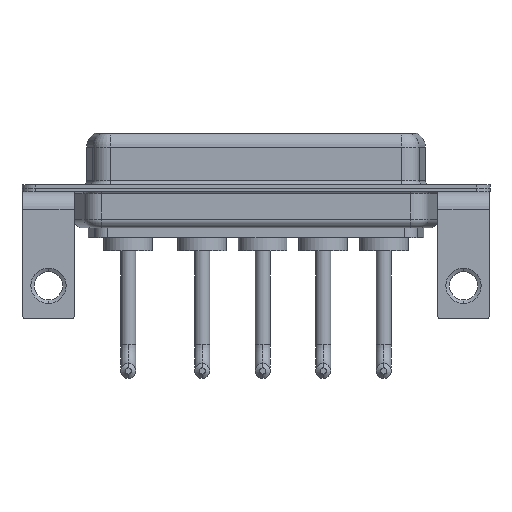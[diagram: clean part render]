
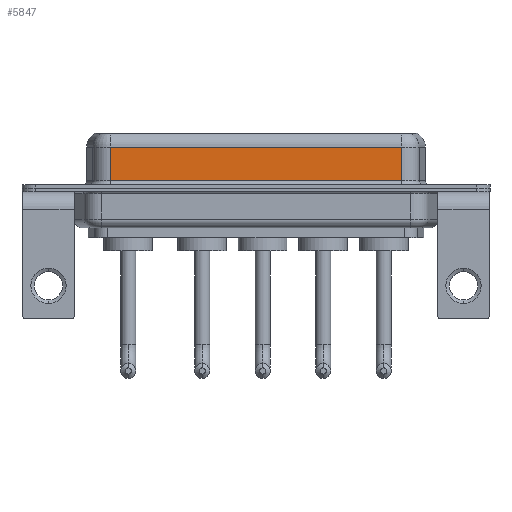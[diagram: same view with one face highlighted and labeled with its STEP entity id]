
A CAD part, front view. The second image highlights one B-rep face of the part: STEP entity #5847.
In plain terms, the highlighted planar face has unit normal (0, -1, 0).
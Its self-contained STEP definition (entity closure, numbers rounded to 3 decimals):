
#731 = CARTESIAN_POINT ( 'NONE',  ( 7.013, -3.95, 6.4 ) ) ;
#1156 = CARTESIAN_POINT ( 'NONE',  ( 40.037, -3.95, 6.4 ) ) ;
#1762 = CARTESIAN_POINT ( 'NONE',  ( 40.037, -3.95, 0.9 ) ) ;
#1887 = VECTOR ( 'NONE', #12253, 1000. ) ;
#1921 = CARTESIAN_POINT ( 'NONE',  ( 40.037, -3.95, 0.9 ) ) ;
#2321 = ORIENTED_EDGE ( 'NONE', *, *, #8391, .T. ) ;
#3272 = ORIENTED_EDGE ( 'NONE', *, *, #5163, .T. ) ;
#3285 = VERTEX_POINT ( 'NONE', #9880 ) ;
#3737 = LINE ( 'NONE', #1762, #1887 ) ;
#3812 = LINE ( 'NONE', #731, #10979 ) ;
#5163 = EDGE_CURVE ( 'NONE', #3285, #8501, #3737, .T. ) ;
#5331 = DIRECTION ( 'NONE',  ( 0., 1., 0. ) ) ;
#5847 = ADVANCED_FACE ( 'NONE', ( #6376 ), #9609, .F. ) ;
#5877 = CARTESIAN_POINT ( 'NONE',  ( 40.037, -3.95, 6.4 ) ) ;
#5925 = ORIENTED_EDGE ( 'NONE', *, *, #10108, .F. ) ;
#6376 = FACE_OUTER_BOUND ( 'NONE', #12402, .T. ) ;
#7046 = LINE ( 'NONE', #10032, #8157 ) ;
#7279 = VERTEX_POINT ( 'NONE', #11904 ) ;
#7931 = DIRECTION ( 'NONE',  ( 0., 0., -1. ) ) ;
#8157 = VECTOR ( 'NONE', #10154, 1000. ) ;
#8391 = EDGE_CURVE ( 'NONE', #7279, #12437, #7046, .T. ) ;
#8501 = VERTEX_POINT ( 'NONE', #1921 ) ;
#8765 = EDGE_CURVE ( 'NONE', #12437, #3285, #3812, .T. ) ;
#9609 = PLANE ( 'NONE',  #10260 ) ;
#9880 = CARTESIAN_POINT ( 'NONE',  ( 7.013, -3.95, 0.9 ) ) ;
#10032 = CARTESIAN_POINT ( 'NONE',  ( 40.037, -3.95, 4.65 ) ) ;
#10108 = EDGE_CURVE ( 'NONE', #7279, #8501, #12197, .T. ) ;
#10154 = DIRECTION ( 'NONE',  ( -1., 0., 0. ) ) ;
#10260 = AXIS2_PLACEMENT_3D ( 'NONE', #1156, #5331, #11597 ) ;
#10979 = VECTOR ( 'NONE', #7931, 1000. ) ;
#11010 = CARTESIAN_POINT ( 'NONE',  ( 7.013, -3.95, 4.65 ) ) ;
#11416 = ORIENTED_EDGE ( 'NONE', *, *, #8765, .T. ) ;
#11597 = DIRECTION ( 'NONE',  ( 0., 0., 1. ) ) ;
#11904 = CARTESIAN_POINT ( 'NONE',  ( 40.037, -3.95, 4.65 ) ) ;
#12104 = VECTOR ( 'NONE', #13147, 1000. ) ;
#12197 = LINE ( 'NONE', #5877, #12104 ) ;
#12253 = DIRECTION ( 'NONE',  ( 1., 0., 0. ) ) ;
#12402 = EDGE_LOOP ( 'NONE', ( #5925, #2321, #11416, #3272 ) ) ;
#12437 = VERTEX_POINT ( 'NONE', #11010 ) ;
#13147 = DIRECTION ( 'NONE',  ( 0., 0., -1. ) ) ;
